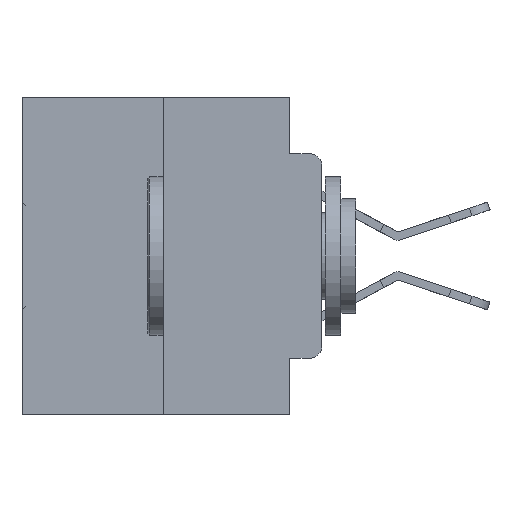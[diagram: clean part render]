
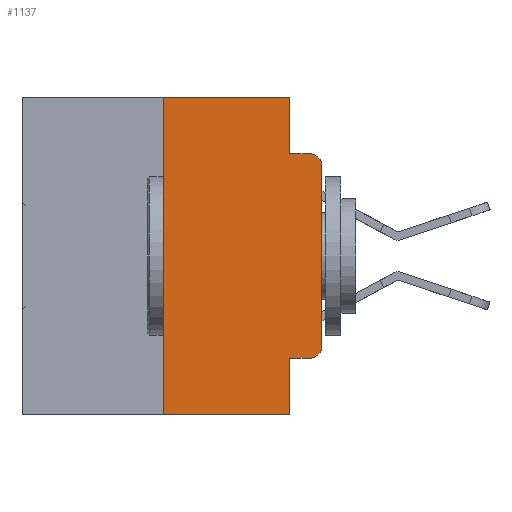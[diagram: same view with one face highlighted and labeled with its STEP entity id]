
A CAD part, left-side view. The second image highlights one B-rep face of the part: STEP entity #1137.
In plain terms, the highlighted planar face has unit normal (-1, 0, 0).
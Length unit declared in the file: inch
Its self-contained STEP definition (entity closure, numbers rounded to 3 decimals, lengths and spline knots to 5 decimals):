
#361 = LINE ( 'NONE', #9999, #26063 ) ;
#680 = DIRECTION ( 'NONE',  ( 0., 0., 1. ) ) ;
#1137 = ADVANCED_FACE ( 'NONE', ( #21199 ), #7742, .F. ) ;
#1485 = DIRECTION ( 'NONE',  ( 0., 0., -1. ) ) ;
#1534 = EDGE_CURVE ( 'NONE', #30027, #14721, #22743, .T. ) ;
#1555 = VECTOR ( 'NONE', #28455, 39.37008 ) ;
#1681 = DIRECTION ( 'NONE',  ( -1., 0., 0. ) ) ;
#1700 = LINE ( 'NONE', #24604, #28420 ) ;
#2444 = CARTESIAN_POINT ( 'NONE',  ( 0., 0.051, -0.4115 ) ) ;
#2500 = DIRECTION ( 'NONE',  ( 0., -1., 0. ) ) ;
#2905 = CARTESIAN_POINT ( 'NONE',  ( 0., 0.473, -0.5 ) ) ;
#3162 = DIRECTION ( 'NONE',  ( -1., 0., 0. ) ) ;
#3168 = VECTOR ( 'NONE', #23951, 39.37008 ) ;
#3877 = LINE ( 'NONE', #2905, #15783 ) ;
#3915 = DIRECTION ( 'NONE',  ( 0., 0., -1. ) ) ;
#4095 = CARTESIAN_POINT ( 'NONE',  ( 0., 0.02, -0.3915 ) ) ;
#4411 = LINE ( 'NONE', #13337, #28726 ) ;
#5258 = EDGE_CURVE ( 'NONE', #8387, #12893, #4411, .T. ) ;
#5633 = CARTESIAN_POINT ( 'NONE',  ( 0., 0.02, -0.0885 ) ) ;
#5899 = DIRECTION ( 'NONE',  ( 0., 0., 1. ) ) ;
#7086 = CARTESIAN_POINT ( 'NONE',  ( 0., 0.02, -0.4115 ) ) ;
#7277 = VERTEX_POINT ( 'NONE', #29207 ) ;
#7433 = ORIENTED_EDGE ( 'NONE', *, *, #1534, .T. ) ;
#7451 = VERTEX_POINT ( 'NONE', #27384 ) ;
#7742 = PLANE ( 'NONE',  #14462 ) ;
#8364 = LINE ( 'NONE', #25993, #1555 ) ;
#8387 = VERTEX_POINT ( 'NONE', #28005 ) ;
#8869 = ORIENTED_EDGE ( 'NONE', *, *, #21634, .F. ) ;
#9563 = DIRECTION ( 'NONE',  ( 0., 0., -1. ) ) ;
#9870 = LINE ( 'NONE', #26343, #3168 ) ;
#9889 = VECTOR ( 'NONE', #30576, 39.37008 ) ;
#9999 = CARTESIAN_POINT ( 'NONE',  ( 0., 0.051, -0.4115 ) ) ;
#10617 = CARTESIAN_POINT ( 'NONE',  ( 0., 0.473, 0. ) ) ;
#11394 = CARTESIAN_POINT ( 'NONE',  ( 0., 0., -0.1085 ) ) ;
#11462 = CARTESIAN_POINT ( 'NONE',  ( 0., 0.25, 0. ) ) ;
#12412 = LINE ( 'NONE', #18490, #17600 ) ;
#12537 = ORIENTED_EDGE ( 'NONE', *, *, #24794, .T. ) ;
#12603 = AXIS2_PLACEMENT_3D ( 'NONE', #18312, #3162, #20809 ) ;
#12893 = VERTEX_POINT ( 'NONE', #11462 ) ;
#13337 = CARTESIAN_POINT ( 'NONE',  ( 0., 0.25, 0. ) ) ;
#14396 = CARTESIAN_POINT ( 'NONE',  ( 0., 0.473, 0. ) ) ;
#14462 = AXIS2_PLACEMENT_3D ( 'NONE', #14396, #15875, #3915 ) ;
#14474 = EDGE_CURVE ( 'NONE', #31879, #30027, #361, .T. ) ;
#14641 = EDGE_CURVE ( 'NONE', #14839, #30347, #27971, .T. ) ;
#14721 = VERTEX_POINT ( 'NONE', #18643 ) ;
#14839 = VERTEX_POINT ( 'NONE', #11394 ) ;
#15367 = EDGE_LOOP ( 'NONE', ( #23638, #23829, #19854, #8869, #16783, #15657, #12537, #17934, #19344, #7433 ) ) ;
#15657 = ORIENTED_EDGE ( 'NONE', *, *, #5258, .F. ) ;
#15783 = VECTOR ( 'NONE', #25564, 39.37008 ) ;
#15875 = DIRECTION ( 'NONE',  ( 1., 0., 0. ) ) ;
#16783 = ORIENTED_EDGE ( 'NONE', *, *, #29176, .F. ) ;
#17451 = LINE ( 'NONE', #10617, #9889 ) ;
#17600 = VECTOR ( 'NONE', #5899, 39.37008 ) ;
#17934 = ORIENTED_EDGE ( 'NONE', *, *, #23833, .F. ) ;
#18312 = CARTESIAN_POINT ( 'NONE',  ( 0., 0.02, -0.1085 ) ) ;
#18490 = CARTESIAN_POINT ( 'NONE',  ( 0., 0., 0. ) ) ;
#18643 = CARTESIAN_POINT ( 'NONE',  ( 0., 0., -0.3915 ) ) ;
#19344 = ORIENTED_EDGE ( 'NONE', *, *, #14474, .T. ) ;
#19854 = ORIENTED_EDGE ( 'NONE', *, *, #29255, .F. ) ;
#20809 = DIRECTION ( 'NONE',  ( 0., 0., -1. ) ) ;
#21199 = FACE_OUTER_BOUND ( 'NONE', #15367, .T. ) ;
#21634 = EDGE_CURVE ( 'NONE', #7451, #7277, #1700, .T. ) ;
#22743 = CIRCLE ( 'NONE', #27190, 0.02 ) ;
#23638 = ORIENTED_EDGE ( 'NONE', *, *, #26296, .T. ) ;
#23829 = ORIENTED_EDGE ( 'NONE', *, *, #14641, .T. ) ;
#23833 = EDGE_CURVE ( 'NONE', #31879, #26441, #9870, .T. ) ;
#23951 = DIRECTION ( 'NONE',  ( 0., 0., -1. ) ) ;
#24604 = CARTESIAN_POINT ( 'NONE',  ( 0., 0.051, 0. ) ) ;
#24794 = EDGE_CURVE ( 'NONE', #8387, #26441, #3877, .T. ) ;
#25564 = DIRECTION ( 'NONE',  ( 0., -1., 0. ) ) ;
#25993 = CARTESIAN_POINT ( 'NONE',  ( 0., 0.051, -0.0885 ) ) ;
#26063 = VECTOR ( 'NONE', #2500, 39.37008 ) ;
#26296 = EDGE_CURVE ( 'NONE', #14721, #14839, #12412, .T. ) ;
#26343 = CARTESIAN_POINT ( 'NONE',  ( 0., 0.051, 0. ) ) ;
#26441 = VERTEX_POINT ( 'NONE', #26481 ) ;
#26481 = CARTESIAN_POINT ( 'NONE',  ( 0., 0.051, -0.5 ) ) ;
#27190 = AXIS2_PLACEMENT_3D ( 'NONE', #4095, #1681, #1485 ) ;
#27384 = CARTESIAN_POINT ( 'NONE',  ( 0., 0.051, 0. ) ) ;
#27971 = CIRCLE ( 'NONE', #12603, 0.02 ) ;
#28005 = CARTESIAN_POINT ( 'NONE',  ( 0., 0.25, -0.5 ) ) ;
#28420 = VECTOR ( 'NONE', #9563, 39.37008 ) ;
#28455 = DIRECTION ( 'NONE',  ( 0., -1., 0. ) ) ;
#28726 = VECTOR ( 'NONE', #680, 39.37008 ) ;
#29176 = EDGE_CURVE ( 'NONE', #12893, #7451, #17451, .T. ) ;
#29207 = CARTESIAN_POINT ( 'NONE',  ( 0., 0.051, -0.0885 ) ) ;
#29255 = EDGE_CURVE ( 'NONE', #7277, #30347, #8364, .T. ) ;
#30027 = VERTEX_POINT ( 'NONE', #7086 ) ;
#30347 = VERTEX_POINT ( 'NONE', #5633 ) ;
#30576 = DIRECTION ( 'NONE',  ( 0., -1., 0. ) ) ;
#31879 = VERTEX_POINT ( 'NONE', #2444 ) ;
